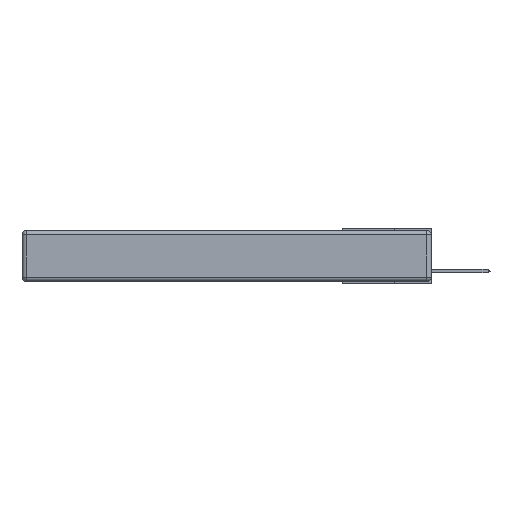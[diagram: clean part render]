
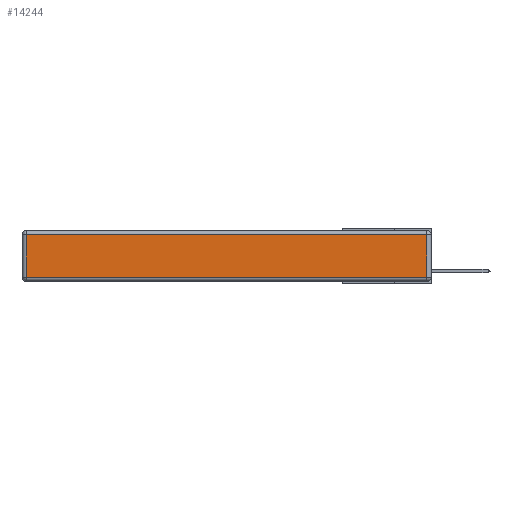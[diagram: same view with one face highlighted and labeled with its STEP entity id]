
A CAD part, left-side view. The second image highlights one B-rep face of the part: STEP entity #14244.
In plain terms, the highlighted planar face has unit normal (-1, 0, 0).
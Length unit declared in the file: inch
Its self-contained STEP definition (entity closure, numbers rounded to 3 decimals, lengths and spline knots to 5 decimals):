
#429 = DIRECTION ( 'NONE',  ( 0., 0., 1. ) ) ;
#614 = CARTESIAN_POINT ( 'NONE',  ( 0., 0.03, -0.343 ) ) ;
#883 = CARTESIAN_POINT ( 'NONE',  ( 0., 0., -0.313 ) ) ;
#1057 = LINE ( 'NONE', #614, #4894 ) ;
#2223 = CARTESIAN_POINT ( 'NONE',  ( 0., 0.03, -0.313 ) ) ;
#2343 = VERTEX_POINT ( 'NONE', #12085 ) ;
#2977 = LINE ( 'NONE', #3977, #5593 ) ;
#3097 = DIRECTION ( 'NONE',  ( 0., -1., 0. ) ) ;
#3178 = EDGE_CURVE ( 'NONE', #11046, #2343, #1057, .T. ) ;
#3270 = FACE_OUTER_BOUND ( 'NONE', #8425, .T. ) ;
#3977 = CARTESIAN_POINT ( 'NONE',  ( 0., 2.75, -0.03 ) ) ;
#4775 = PLANE ( 'NONE',  #10962 ) ;
#4885 = ORIENTED_EDGE ( 'NONE', *, *, #3178, .T. ) ;
#4894 = VECTOR ( 'NONE', #8358, 39.37008 ) ;
#5468 = EDGE_CURVE ( 'NONE', #9328, #8108, #8073, .T. ) ;
#5593 = VECTOR ( 'NONE', #13009, 39.37008 ) ;
#6747 = CARTESIAN_POINT ( 'NONE',  ( 0., 2.72, -0.313 ) ) ;
#7041 = ORIENTED_EDGE ( 'NONE', *, *, #11207, .T. ) ;
#7055 = DIRECTION ( 'NONE',  ( -1., 0., 0. ) ) ;
#8025 = CARTESIAN_POINT ( 'NONE',  ( 0., 0., -0.343 ) ) ;
#8073 = LINE ( 'NONE', #14110, #10702 ) ;
#8108 = VERTEX_POINT ( 'NONE', #6747 ) ;
#8358 = DIRECTION ( 'NONE',  ( 0., 0., 1. ) ) ;
#8425 = EDGE_LOOP ( 'NONE', ( #14055, #4885, #7041, #8992 ) ) ;
#8992 = ORIENTED_EDGE ( 'NONE', *, *, #5468, .T. ) ;
#9328 = VERTEX_POINT ( 'NONE', #9520 ) ;
#9520 = CARTESIAN_POINT ( 'NONE',  ( 0., 2.72, -0.03 ) ) ;
#9739 = LINE ( 'NONE', #883, #12713 ) ;
#10667 = DIRECTION ( 'NONE',  ( 0., 0., -1. ) ) ;
#10702 = VECTOR ( 'NONE', #10667, 39.37008 ) ;
#10962 = AXIS2_PLACEMENT_3D ( 'NONE', #8025, #7055, #429 ) ;
#11046 = VERTEX_POINT ( 'NONE', #2223 ) ;
#11207 = EDGE_CURVE ( 'NONE', #2343, #9328, #2977, .T. ) ;
#12085 = CARTESIAN_POINT ( 'NONE',  ( 0., 0.03, -0.03 ) ) ;
#12713 = VECTOR ( 'NONE', #3097, 39.37008 ) ;
#13009 = DIRECTION ( 'NONE',  ( 0., 1., 0. ) ) ;
#13166 = EDGE_CURVE ( 'NONE', #8108, #11046, #9739, .T. ) ;
#14055 = ORIENTED_EDGE ( 'NONE', *, *, #13166, .T. ) ;
#14110 = CARTESIAN_POINT ( 'NONE',  ( 0., 2.72, -0.343 ) ) ;
#14244 = ADVANCED_FACE ( 'NONE', ( #3270 ), #4775, .T. ) ;
